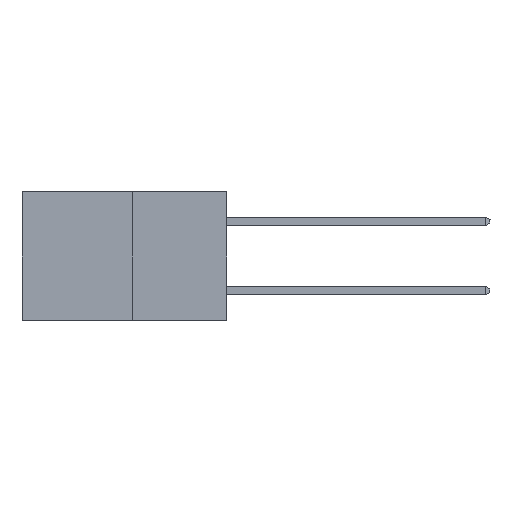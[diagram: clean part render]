
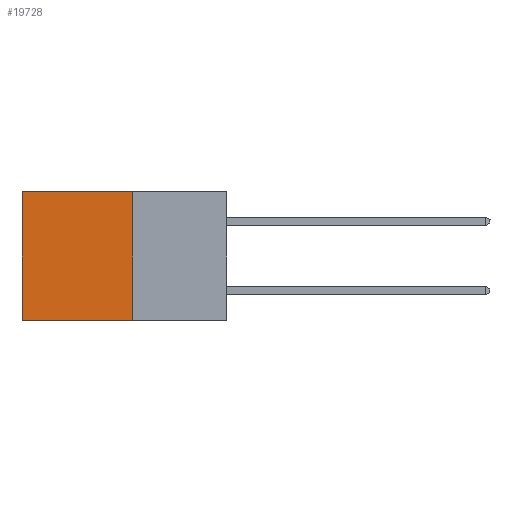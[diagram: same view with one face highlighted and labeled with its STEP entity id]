
A CAD part, left-side view. The second image highlights one B-rep face of the part: STEP entity #19728.
In plain terms, the highlighted planar face has unit normal (-1, 0, 0).
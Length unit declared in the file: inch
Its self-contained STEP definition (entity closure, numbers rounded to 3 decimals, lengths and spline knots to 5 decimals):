
#22 = EDGE_CURVE ( 'NONE', #13595, #5938, #22899, .T. ) ;
#1135 = CARTESIAN_POINT ( 'NONE',  ( 0.277, 0.27, 0. ) ) ;
#1481 = EDGE_CURVE ( 'NONE', #16778, #27857, #11279, .T. ) ;
#1809 = EDGE_CURVE ( 'NONE', #5938, #27857, #8259, .T. ) ;
#5396 = EDGE_LOOP ( 'NONE', ( #11213, #17387, #7290, #34356 ) ) ;
#5938 = VERTEX_POINT ( 'NONE', #11646 ) ;
#7290 = ORIENTED_EDGE ( 'NONE', *, *, #22, .F. ) ;
#8259 = LINE ( 'NONE', #18643, #29106 ) ;
#11213 = ORIENTED_EDGE ( 'NONE', *, *, #1481, .T. ) ;
#11279 = LINE ( 'NONE', #21147, #32057 ) ;
#11646 = CARTESIAN_POINT ( 'NONE',  ( 0.277, 0.27, -0.37 ) ) ;
#13595 = VERTEX_POINT ( 'NONE', #33809 ) ;
#13788 = PLANE ( 'NONE',  #31307 ) ;
#14176 = DIRECTION ( 'NONE',  ( 0., 1., 0. ) ) ;
#16255 = DIRECTION ( 'NONE',  ( 0., 0., -1. ) ) ;
#16541 = DIRECTION ( 'NONE',  ( 0., 0., -1. ) ) ;
#16778 = VERTEX_POINT ( 'NONE', #34133 ) ;
#17387 = ORIENTED_EDGE ( 'NONE', *, *, #1809, .F. ) ;
#17806 = EDGE_CURVE ( 'NONE', #13595, #16778, #24749, .T. ) ;
#18643 = CARTESIAN_POINT ( 'NONE',  ( 0.277, 0.27, -0.37 ) ) ;
#19728 = ADVANCED_FACE ( 'NONE', ( #19749 ), #13788, .F. ) ;
#19749 = FACE_OUTER_BOUND ( 'NONE', #5396, .T. ) ;
#21147 = CARTESIAN_POINT ( 'NONE',  ( 0.277, 0.59, -0.37 ) ) ;
#21953 = CARTESIAN_POINT ( 'NONE',  ( 0.277, 0.27, -0.37 ) ) ;
#22314 = CARTESIAN_POINT ( 'NONE',  ( 0.277, 0.59, -0.37 ) ) ;
#22899 = LINE ( 'NONE', #30773, #23780 ) ;
#23061 = VECTOR ( 'NONE', #31135, 39.37008 ) ;
#23313 = DIRECTION ( 'NONE',  ( 0., 0., -1. ) ) ;
#23780 = VECTOR ( 'NONE', #16255, 39.37008 ) ;
#24749 = LINE ( 'NONE', #1135, #23061 ) ;
#27857 = VERTEX_POINT ( 'NONE', #22314 ) ;
#29106 = VECTOR ( 'NONE', #14176, 39.37008 ) ;
#30773 = CARTESIAN_POINT ( 'NONE',  ( 0.277, 0.27, -0.37 ) ) ;
#31135 = DIRECTION ( 'NONE',  ( 0., 1., 0. ) ) ;
#31307 = AXIS2_PLACEMENT_3D ( 'NONE', #21953, #32770, #16541 ) ;
#32057 = VECTOR ( 'NONE', #23313, 39.37008 ) ;
#32770 = DIRECTION ( 'NONE',  ( 1., 0., 0. ) ) ;
#33809 = CARTESIAN_POINT ( 'NONE',  ( 0.277, 0.27, 0. ) ) ;
#34133 = CARTESIAN_POINT ( 'NONE',  ( 0.277, 0.59, 0. ) ) ;
#34356 = ORIENTED_EDGE ( 'NONE', *, *, #17806, .T. ) ;
